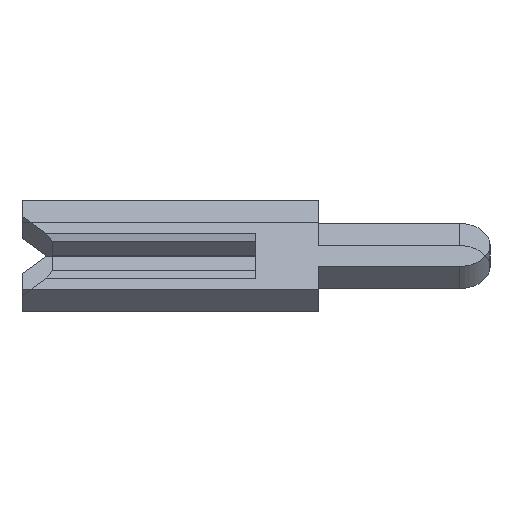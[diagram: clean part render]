
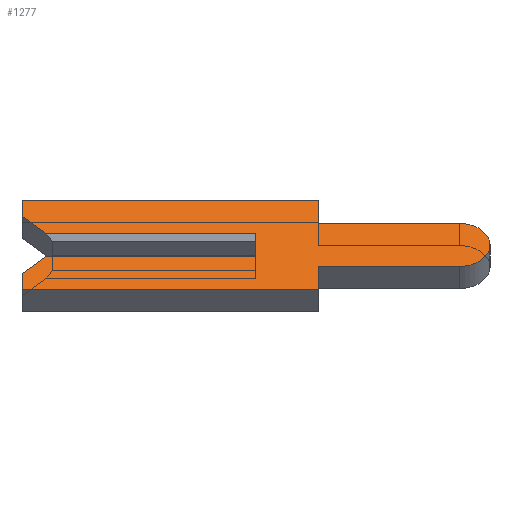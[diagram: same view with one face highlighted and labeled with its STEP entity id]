
A CAD part, left-side view. The second image highlights one B-rep face of the part: STEP entity #1277.
In plain terms, the highlighted face is planar.
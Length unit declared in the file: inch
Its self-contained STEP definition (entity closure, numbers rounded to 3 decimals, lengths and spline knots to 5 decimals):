
#25 = LINE ( 'NONE', #1379, #1316 ) ;
#26 = VERTEX_POINT ( 'NONE', #1750 ) ;
#43 = DIRECTION ( 'NONE',  ( 0., 0., -1. ) ) ;
#47 = ORIENTED_EDGE ( 'NONE', *, *, #1506, .F. ) ;
#51 = CARTESIAN_POINT ( 'NONE',  ( -0.01, 0.1305, -0.0065 ) ) ;
#56 = LINE ( 'NONE', #1857, #928 ) ;
#73 = AXIS2_PLACEMENT_3D ( 'NONE', #1975, #1009, #43 ) ;
#82 = VERTEX_POINT ( 'NONE', #934 ) ;
#96 = LINE ( 'NONE', #1085, #1358 ) ;
#97 = EDGE_CURVE ( 'NONE', #82, #1960, #96, .T. ) ;
#118 = CARTESIAN_POINT ( 'NONE',  ( -0.01, -0.04, 0.0195 ) ) ;
#119 = VECTOR ( 'NONE', #261, 39.37008 ) ;
#148 = VECTOR ( 'NONE', #626, 39.37008 ) ;
#152 = VECTOR ( 'NONE', #1184, 39.37008 ) ;
#185 = EDGE_CURVE ( 'NONE', #725, #1893, #683, .T. ) ;
#195 = ORIENTED_EDGE ( 'NONE', *, *, #1271, .F. ) ;
#196 = DIRECTION ( 'NONE',  ( 0., 1., 0. ) ) ;
#235 = DIRECTION ( 'NONE',  ( 0., -1., 0. ) ) ;
#244 = DIRECTION ( 'NONE',  ( 0., -0.707, 0.707 ) ) ;
#245 = VERTEX_POINT ( 'NONE', #300 ) ;
#261 = DIRECTION ( 'NONE',  ( 0., 1., 0. ) ) ;
#276 = DIRECTION ( 'NONE',  ( 0., 0., -1. ) ) ;
#282 = CARTESIAN_POINT ( 'NONE',  ( -0.01, -0.04, 0.0195 ) ) ;
#283 = ORIENTED_EDGE ( 'NONE', *, *, #1600, .F. ) ;
#300 = CARTESIAN_POINT ( 'NONE',  ( -0.01, 0., 0.01 ) ) ;
#378 = VECTOR ( 'NONE', #2015, 39.37008 ) ;
#396 = CARTESIAN_POINT ( 'NONE',  ( -0.01, 0.134, 0.01 ) ) ;
#420 = LINE ( 'NONE', #884, #2032 ) ;
#437 = ORIENTED_EDGE ( 'NONE', *, *, #987, .F. ) ;
#446 = ORIENTED_EDGE ( 'NONE', *, *, #97, .F. ) ;
#461 = VERTEX_POINT ( 'NONE', #468 ) ;
#468 = CARTESIAN_POINT ( 'NONE',  ( -0.01, 0.15, 0.04 ) ) ;
#473 = VERTEX_POINT ( 'NONE', #963 ) ;
#538 = DIRECTION ( 'NONE',  ( 0., 0., 1. ) ) ;
#547 = ORIENTED_EDGE ( 'NONE', *, *, #185, .F. ) ;
#557 = VECTOR ( 'NONE', #235, 39.37008 ) ;
#603 = CIRCLE ( 'NONE', #73, 0.0195 ) ;
#626 = DIRECTION ( 'NONE',  ( 0., -1., 0. ) ) ;
#683 = LINE ( 'NONE', #118, #148 ) ;
#725 = VERTEX_POINT ( 'NONE', #282 ) ;
#755 = CARTESIAN_POINT ( 'NONE',  ( -0.01, -0.1305, -0.01 ) ) ;
#779 = LINE ( 'NONE', #755, #378 ) ;
#824 = ORIENTED_EDGE ( 'NONE', *, *, #1573, .F. ) ;
#832 = VECTOR ( 'NONE', #1368, 39.37008 ) ;
#853 = ORIENTED_EDGE ( 'NONE', *, *, #861, .F. ) ;
#861 = EDGE_CURVE ( 'NONE', #1960, #1025, #1528, .T. ) ;
#864 = CARTESIAN_POINT ( 'NONE',  ( -0.01, -0.1305, 0. ) ) ;
#869 = CARTESIAN_POINT ( 'NONE',  ( -0.01, 0.15, -0.026 ) ) ;
#884 = CARTESIAN_POINT ( 'NONE',  ( -0.01, 0.15, 0.01 ) ) ;
#890 = CARTESIAN_POINT ( 'NONE',  ( -0.01, 0.134, -0.01 ) ) ;
#916 = ORIENTED_EDGE ( 'NONE', *, *, #1186, .F. ) ;
#928 = VECTOR ( 'NONE', #1218, 39.37008 ) ;
#934 = CARTESIAN_POINT ( 'NONE',  ( -0.01, -0.04, -0.0195 ) ) ;
#963 = CARTESIAN_POINT ( 'NONE',  ( -0.01, 0., -0.01 ) ) ;
#987 = EDGE_CURVE ( 'NONE', #1347, #725, #1081, .T. ) ;
#1001 = LINE ( 'NONE', #51, #1863 ) ;
#1009 = DIRECTION ( 'NONE',  ( 1., 0., 0. ) ) ;
#1025 = VERTEX_POINT ( 'NONE', #1953 ) ;
#1050 = AXIS2_PLACEMENT_3D ( 'NONE', #864, #1204, #1692 ) ;
#1058 = CARTESIAN_POINT ( 'NONE',  ( -0.01, -0.04, -0.0195 ) ) ;
#1068 = CARTESIAN_POINT ( 'NONE',  ( -0.01, 0.15, 0.026 ) ) ;
#1074 = VECTOR ( 'NONE', #196, 39.37008 ) ;
#1081 = LINE ( 'NONE', #1517, #1999 ) ;
#1085 = CARTESIAN_POINT ( 'NONE',  ( -0.01, -0.04, -0.04 ) ) ;
#1090 = LINE ( 'NONE', #1840, #832 ) ;
#1101 = EDGE_CURVE ( 'NONE', #1893, #26, #603, .T. ) ;
#1155 = ORIENTED_EDGE ( 'NONE', *, *, #1101, .F. ) ;
#1184 = DIRECTION ( 'NONE',  ( 0., 0.707, 0.707 ) ) ;
#1186 = EDGE_CURVE ( 'NONE', #1279, #1717, #1303, .T. ) ;
#1201 = EDGE_CURVE ( 'NONE', #1025, #1317, #25, .T. ) ;
#1204 = DIRECTION ( 'NONE',  ( 1., 0., 0. ) ) ;
#1213 = EDGE_CURVE ( 'NONE', #1317, #1969, #1001, .T. ) ;
#1218 = DIRECTION ( 'NONE',  ( 0., 0., 1. ) ) ;
#1252 = EDGE_CURVE ( 'NONE', #1717, #461, #1090, .T. ) ;
#1271 = EDGE_CURVE ( 'NONE', #461, #1347, #1773, .T. ) ;
#1277 = ADVANCED_FACE ( 'NONE', ( #1386 ), #1826, .F. ) ;
#1279 = VERTEX_POINT ( 'NONE', #396 ) ;
#1303 = LINE ( 'NONE', #1391, #152 ) ;
#1316 = VECTOR ( 'NONE', #538, 39.37008 ) ;
#1317 = VERTEX_POINT ( 'NONE', #869 ) ;
#1334 = CARTESIAN_POINT ( 'NONE',  ( -0.01, 0.15, -0.04 ) ) ;
#1347 = VERTEX_POINT ( 'NONE', #2006 ) ;
#1355 = EDGE_CURVE ( 'NONE', #1279, #245, #420, .T. ) ;
#1358 = VECTOR ( 'NONE', #276, 39.37008 ) ;
#1368 = DIRECTION ( 'NONE',  ( 0., 0., 1. ) ) ;
#1372 = ORIENTED_EDGE ( 'NONE', *, *, #1201, .F. ) ;
#1379 = CARTESIAN_POINT ( 'NONE',  ( -0.01, 0.15, -0.026 ) ) ;
#1386 = FACE_OUTER_BOUND ( 'NONE', #1902, .T. ) ;
#1387 = CARTESIAN_POINT ( 'NONE',  ( -0.01, 0.15, 0.04 ) ) ;
#1391 = CARTESIAN_POINT ( 'NONE',  ( -0.01, 0.1305, 0.0065 ) ) ;
#1506 = EDGE_CURVE ( 'NONE', #1969, #473, #779, .T. ) ;
#1517 = CARTESIAN_POINT ( 'NONE',  ( -0.01, -0.04, 0.04 ) ) ;
#1528 = LINE ( 'NONE', #1334, #1074 ) ;
#1533 = DIRECTION ( 'NONE',  ( 0., -1., 0. ) ) ;
#1546 = ORIENTED_EDGE ( 'NONE', *, *, #1355, .T. ) ;
#1573 = EDGE_CURVE ( 'NONE', #26, #82, #1620, .T. ) ;
#1576 = CARTESIAN_POINT ( 'NONE',  ( -0.01, -0.04, -0.04 ) ) ;
#1600 = EDGE_CURVE ( 'NONE', #473, #245, #56, .T. ) ;
#1620 = LINE ( 'NONE', #1058, #119 ) ;
#1640 = DIRECTION ( 'NONE',  ( 0., 0., -1. ) ) ;
#1692 = DIRECTION ( 'NONE',  ( 0., 0., -1. ) ) ;
#1717 = VERTEX_POINT ( 'NONE', #1068 ) ;
#1750 = CARTESIAN_POINT ( 'NONE',  ( -0.01, -0.1305, -0.0195 ) ) ;
#1773 = LINE ( 'NONE', #1387, #557 ) ;
#1826 = PLANE ( 'NONE',  #1050 ) ;
#1829 = ORIENTED_EDGE ( 'NONE', *, *, #1252, .F. ) ;
#1840 = CARTESIAN_POINT ( 'NONE',  ( -0.01, 0.15, 0.026 ) ) ;
#1857 = CARTESIAN_POINT ( 'NONE',  ( -0.01, 0., 0.0065 ) ) ;
#1863 = VECTOR ( 'NONE', #244, 39.37008 ) ;
#1882 = CARTESIAN_POINT ( 'NONE',  ( -0.01, -0.1305, 0.0195 ) ) ;
#1893 = VERTEX_POINT ( 'NONE', #1882 ) ;
#1897 = ORIENTED_EDGE ( 'NONE', *, *, #1213, .F. ) ;
#1902 = EDGE_LOOP ( 'NONE', ( #1546, #283, #47, #1897, #1372, #853, #446, #824, #1155, #547, #437, #195, #1829, #916 ) ) ;
#1953 = CARTESIAN_POINT ( 'NONE',  ( -0.01, 0.15, -0.04 ) ) ;
#1960 = VERTEX_POINT ( 'NONE', #1576 ) ;
#1969 = VERTEX_POINT ( 'NONE', #890 ) ;
#1975 = CARTESIAN_POINT ( 'NONE',  ( -0.01, -0.1305, 0. ) ) ;
#1999 = VECTOR ( 'NONE', #1640, 39.37008 ) ;
#2006 = CARTESIAN_POINT ( 'NONE',  ( -0.01, -0.04, 0.04 ) ) ;
#2015 = DIRECTION ( 'NONE',  ( 0., -1., 0. ) ) ;
#2032 = VECTOR ( 'NONE', #1533, 39.37008 ) ;
